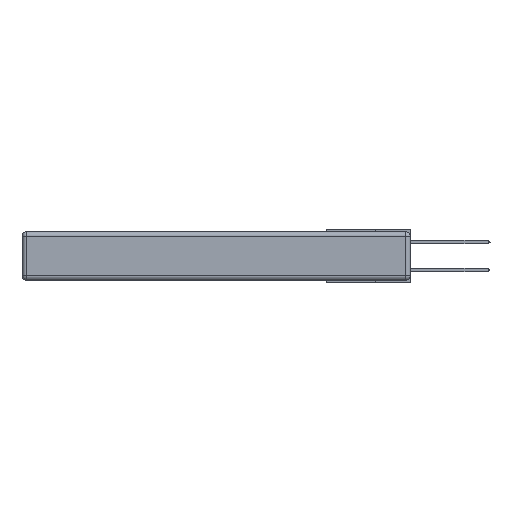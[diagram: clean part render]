
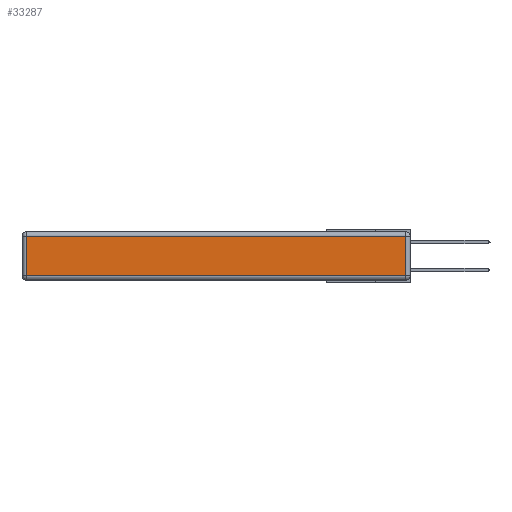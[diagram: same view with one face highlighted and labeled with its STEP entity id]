
A CAD part, left-side view. The second image highlights one B-rep face of the part: STEP entity #33287.
In plain terms, the highlighted planar face has unit normal (-1, 0, 0).
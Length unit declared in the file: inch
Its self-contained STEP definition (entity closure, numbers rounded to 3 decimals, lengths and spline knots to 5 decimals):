
#138 = ORIENTED_EDGE ( 'NONE', *, *, #33573, .T. ) ;
#580 = CARTESIAN_POINT ( 'NONE',  ( 0., 2.75, -0.03 ) ) ;
#1276 = EDGE_CURVE ( 'NONE', #32940, #13161, #12267, .T. ) ;
#2290 = DIRECTION ( 'NONE',  ( 0., 0., -1. ) ) ;
#4091 = VERTEX_POINT ( 'NONE', #28748 ) ;
#4880 = PLANE ( 'NONE',  #13539 ) ;
#6057 = DIRECTION ( 'NONE',  ( 0., 1., 0. ) ) ;
#10288 = CARTESIAN_POINT ( 'NONE',  ( 0., 0., -0.343 ) ) ;
#10313 = LINE ( 'NONE', #29852, #17034 ) ;
#10414 = LINE ( 'NONE', #24790, #15032 ) ;
#11284 = ORIENTED_EDGE ( 'NONE', *, *, #14300, .T. ) ;
#12267 = LINE ( 'NONE', #580, #34049 ) ;
#13161 = VERTEX_POINT ( 'NONE', #19721 ) ;
#13539 = AXIS2_PLACEMENT_3D ( 'NONE', #10288, #17879, #25992 ) ;
#14085 = EDGE_LOOP ( 'NONE', ( #138, #32751, #28141, #11284 ) ) ;
#14300 = EDGE_CURVE ( 'NONE', #13161, #4091, #30704, .T. ) ;
#15032 = VECTOR ( 'NONE', #30220, 39.37008 ) ;
#17034 = VECTOR ( 'NONE', #32925, 39.37008 ) ;
#17385 = VERTEX_POINT ( 'NONE', #28069 ) ;
#17879 = DIRECTION ( 'NONE',  ( -1., 0., 0. ) ) ;
#19721 = CARTESIAN_POINT ( 'NONE',  ( 0., 2.72, -0.03 ) ) ;
#20035 = FACE_OUTER_BOUND ( 'NONE', #14085, .T. ) ;
#23822 = CARTESIAN_POINT ( 'NONE',  ( 0., 2.72, -0.343 ) ) ;
#23874 = EDGE_CURVE ( 'NONE', #17385, #32940, #10414, .T. ) ;
#24790 = CARTESIAN_POINT ( 'NONE',  ( 0., 0.03, -0.343 ) ) ;
#25992 = DIRECTION ( 'NONE',  ( 0., 0., 1. ) ) ;
#27543 = CARTESIAN_POINT ( 'NONE',  ( 0., 0.03, -0.03 ) ) ;
#28069 = CARTESIAN_POINT ( 'NONE',  ( 0., 0.03, -0.313 ) ) ;
#28141 = ORIENTED_EDGE ( 'NONE', *, *, #1276, .T. ) ;
#28748 = CARTESIAN_POINT ( 'NONE',  ( 0., 2.72, -0.313 ) ) ;
#28984 = VECTOR ( 'NONE', #2290, 39.37008 ) ;
#29852 = CARTESIAN_POINT ( 'NONE',  ( 0., 0., -0.313 ) ) ;
#30220 = DIRECTION ( 'NONE',  ( 0., 0., 1. ) ) ;
#30704 = LINE ( 'NONE', #23822, #28984 ) ;
#32751 = ORIENTED_EDGE ( 'NONE', *, *, #23874, .T. ) ;
#32925 = DIRECTION ( 'NONE',  ( 0., -1., 0. ) ) ;
#32940 = VERTEX_POINT ( 'NONE', #27543 ) ;
#33287 = ADVANCED_FACE ( 'NONE', ( #20035 ), #4880, .T. ) ;
#33573 = EDGE_CURVE ( 'NONE', #4091, #17385, #10313, .T. ) ;
#34049 = VECTOR ( 'NONE', #6057, 39.37008 ) ;
